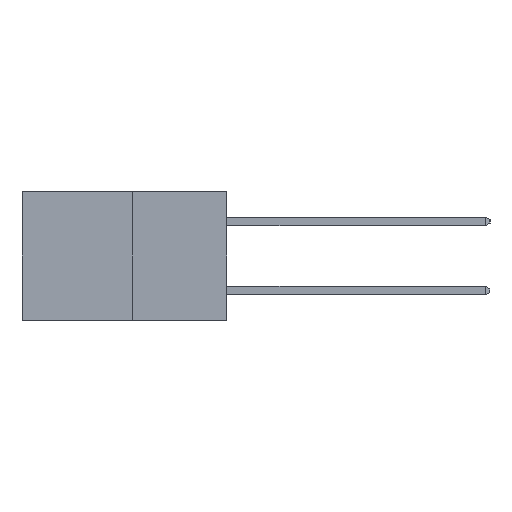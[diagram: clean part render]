
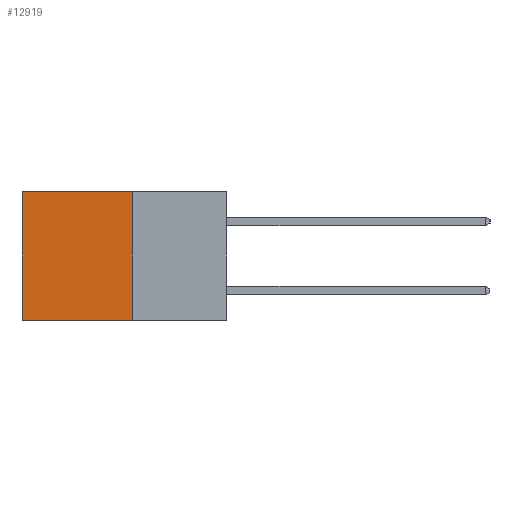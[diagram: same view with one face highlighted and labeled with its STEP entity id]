
A CAD part, left-side view. The second image highlights one B-rep face of the part: STEP entity #12919.
In plain terms, the highlighted planar face has unit normal (-1, 0, 0).
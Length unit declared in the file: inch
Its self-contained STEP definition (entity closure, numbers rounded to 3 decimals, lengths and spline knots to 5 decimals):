
#157 = CARTESIAN_POINT ( 'NONE',  ( 0.277, 0.27, -0.37 ) ) ;
#330 = AXIS2_PLACEMENT_3D ( 'NONE', #11787, #13050, #5618 ) ;
#661 = VECTOR ( 'NONE', #2094, 39.37008 ) ;
#2052 = VECTOR ( 'NONE', #11944, 39.37008 ) ;
#2094 = DIRECTION ( 'NONE',  ( 0., 0., -1. ) ) ;
#2423 = LINE ( 'NONE', #10719, #2052 ) ;
#2907 = LINE ( 'NONE', #13822, #9485 ) ;
#3148 = PLANE ( 'NONE',  #330 ) ;
#3535 = ORIENTED_EDGE ( 'NONE', *, *, #8787, .T. ) ;
#4380 = DIRECTION ( 'NONE',  ( 0., 1., 0. ) ) ;
#5158 = DIRECTION ( 'NONE',  ( 0., 0., -1. ) ) ;
#5618 = DIRECTION ( 'NONE',  ( 0., 0., -1. ) ) ;
#8408 = CARTESIAN_POINT ( 'NONE',  ( 0.277, 0.59, 0. ) ) ;
#8787 = EDGE_CURVE ( 'NONE', #15928, #14308, #13776, .T. ) ;
#9082 = EDGE_CURVE ( 'NONE', #11852, #13994, #2907, .T. ) ;
#9485 = VECTOR ( 'NONE', #5158, 39.37008 ) ;
#10059 = EDGE_CURVE ( 'NONE', #11852, #15928, #15474, .T. ) ;
#10182 = FACE_OUTER_BOUND ( 'NONE', #12714, .T. ) ;
#10517 = CARTESIAN_POINT ( 'NONE',  ( 0.277, 0.59, -0.37 ) ) ;
#10719 = CARTESIAN_POINT ( 'NONE',  ( 0.277, 0.27, -0.37 ) ) ;
#11268 = ORIENTED_EDGE ( 'NONE', *, *, #9082, .F. ) ;
#11787 = CARTESIAN_POINT ( 'NONE',  ( 0.277, 0.27, -0.37 ) ) ;
#11852 = VERTEX_POINT ( 'NONE', #15129 ) ;
#11944 = DIRECTION ( 'NONE',  ( 0., 1., 0. ) ) ;
#12183 = VECTOR ( 'NONE', #4380, 39.37008 ) ;
#12714 = EDGE_LOOP ( 'NONE', ( #3535, #14621, #11268, #15779 ) ) ;
#12919 = ADVANCED_FACE ( 'NONE', ( #10182 ), #3148, .F. ) ;
#13004 = EDGE_CURVE ( 'NONE', #13994, #14308, #2423, .T. ) ;
#13031 = CARTESIAN_POINT ( 'NONE',  ( 0.277, 0.27, 0. ) ) ;
#13050 = DIRECTION ( 'NONE',  ( 1., 0., 0. ) ) ;
#13239 = CARTESIAN_POINT ( 'NONE',  ( 0.277, 0.59, -0.37 ) ) ;
#13776 = LINE ( 'NONE', #13239, #661 ) ;
#13822 = CARTESIAN_POINT ( 'NONE',  ( 0.277, 0.27, -0.37 ) ) ;
#13994 = VERTEX_POINT ( 'NONE', #157 ) ;
#14308 = VERTEX_POINT ( 'NONE', #10517 ) ;
#14621 = ORIENTED_EDGE ( 'NONE', *, *, #13004, .F. ) ;
#15129 = CARTESIAN_POINT ( 'NONE',  ( 0.277, 0.27, 0. ) ) ;
#15474 = LINE ( 'NONE', #13031, #12183 ) ;
#15779 = ORIENTED_EDGE ( 'NONE', *, *, #10059, .T. ) ;
#15928 = VERTEX_POINT ( 'NONE', #8408 ) ;
